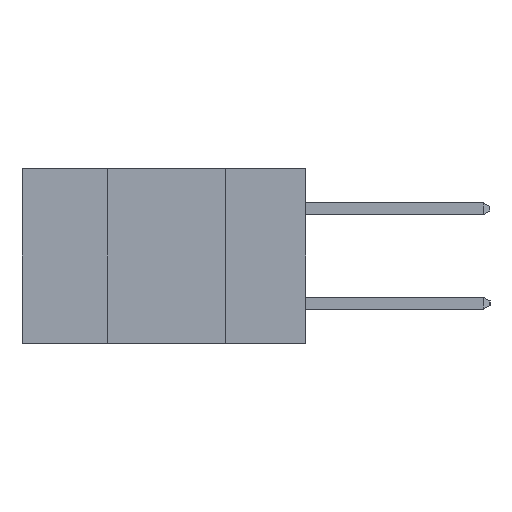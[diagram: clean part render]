
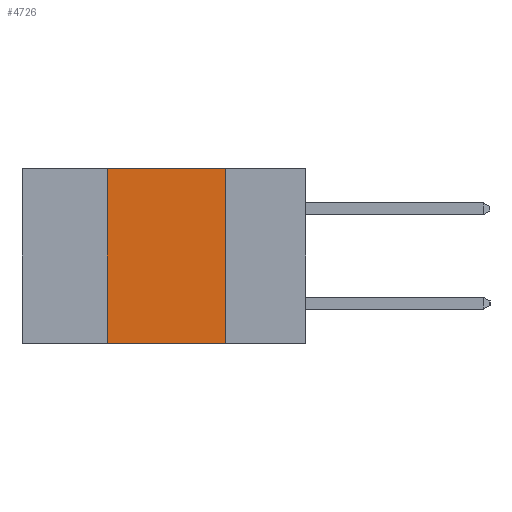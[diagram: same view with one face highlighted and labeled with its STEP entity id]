
A CAD part, left-side view. The second image highlights one B-rep face of the part: STEP entity #4726.
In plain terms, the highlighted planar face has unit normal (-1, 0, 0).
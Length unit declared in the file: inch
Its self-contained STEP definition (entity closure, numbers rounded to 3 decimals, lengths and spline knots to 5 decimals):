
#118 = VECTOR ( 'NONE', #173, 39.37008 ) ;
#173 = DIRECTION ( 'NONE',  ( 0., -1., 0. ) ) ;
#313 = DIRECTION ( 'NONE',  ( 0., 0., -1. ) ) ;
#985 = ORIENTED_EDGE ( 'NONE', *, *, #9684, .F. ) ;
#1095 = CARTESIAN_POINT ( 'NONE',  ( 0., 0.17, -0.37 ) ) ;
#1290 = EDGE_CURVE ( 'NONE', #4413, #3597, #4854, .T. ) ;
#1500 = PLANE ( 'NONE',  #4435 ) ;
#1557 = VECTOR ( 'NONE', #6103, 39.37008 ) ;
#2162 = FACE_OUTER_BOUND ( 'NONE', #9026, .T. ) ;
#2436 = ORIENTED_EDGE ( 'NONE', *, *, #7088, .F. ) ;
#2546 = CARTESIAN_POINT ( 'NONE',  ( 0., 0.42, 0. ) ) ;
#3597 = VERTEX_POINT ( 'NONE', #1095 ) ;
#4141 = CARTESIAN_POINT ( 'NONE',  ( 0., 0.17, 0. ) ) ;
#4413 = VERTEX_POINT ( 'NONE', #4464 ) ;
#4435 = AXIS2_PLACEMENT_3D ( 'NONE', #9441, #4838, #10211 ) ;
#4464 = CARTESIAN_POINT ( 'NONE',  ( 0., 0.42, -0.37 ) ) ;
#4470 = CARTESIAN_POINT ( 'NONE',  ( 0., 0.17, -0.37 ) ) ;
#4590 = CARTESIAN_POINT ( 'NONE',  ( 0., 0.6, -0.37 ) ) ;
#4637 = EDGE_CURVE ( 'NONE', #6143, #5561, #6989, .T. ) ;
#4726 = ADVANCED_FACE ( 'NONE', ( #2162 ), #1500, .F. ) ;
#4838 = DIRECTION ( 'NONE',  ( 1., 0., 0. ) ) ;
#4854 = LINE ( 'NONE', #4590, #118 ) ;
#4908 = VECTOR ( 'NONE', #7100, 39.37008 ) ;
#5117 = LINE ( 'NONE', #4470, #9424 ) ;
#5405 = ORIENTED_EDGE ( 'NONE', *, *, #4637, .F. ) ;
#5561 = VERTEX_POINT ( 'NONE', #4141 ) ;
#5911 = LINE ( 'NONE', #9902, #1557 ) ;
#6103 = DIRECTION ( 'NONE',  ( 0., 0., 1. ) ) ;
#6143 = VERTEX_POINT ( 'NONE', #2546 ) ;
#6989 = LINE ( 'NONE', #8603, #4908 ) ;
#6990 = ORIENTED_EDGE ( 'NONE', *, *, #1290, .T. ) ;
#7088 = EDGE_CURVE ( 'NONE', #5561, #3597, #5117, .T. ) ;
#7100 = DIRECTION ( 'NONE',  ( 0., -1., 0. ) ) ;
#8603 = CARTESIAN_POINT ( 'NONE',  ( 0., 0.6, 0. ) ) ;
#9026 = EDGE_LOOP ( 'NONE', ( #2436, #5405, #985, #6990 ) ) ;
#9424 = VECTOR ( 'NONE', #313, 39.37008 ) ;
#9441 = CARTESIAN_POINT ( 'NONE',  ( 0., 0.6, 0. ) ) ;
#9684 = EDGE_CURVE ( 'NONE', #4413, #6143, #5911, .T. ) ;
#9902 = CARTESIAN_POINT ( 'NONE',  ( 0., 0.42, -0.37 ) ) ;
#10211 = DIRECTION ( 'NONE',  ( 0., 0., -1. ) ) ;
